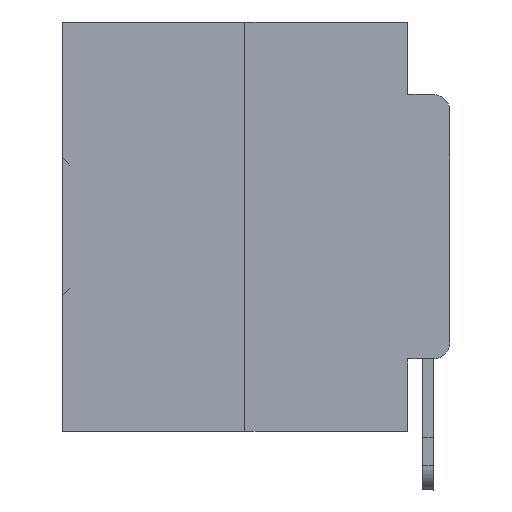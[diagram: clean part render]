
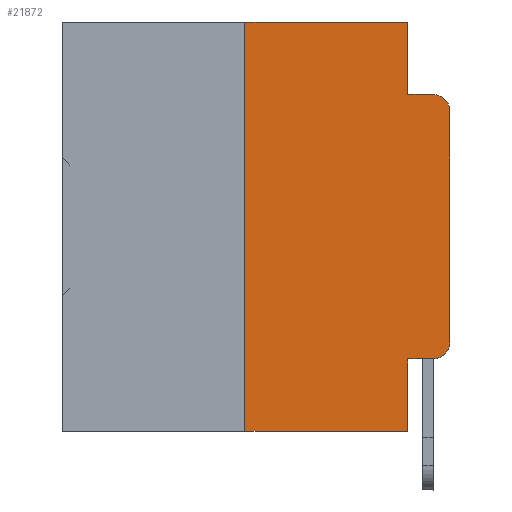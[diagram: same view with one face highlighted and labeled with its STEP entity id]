
A CAD part, left-side view. The second image highlights one B-rep face of the part: STEP entity #21872.
In plain terms, the highlighted planar face has unit normal (-1, 0, 0).
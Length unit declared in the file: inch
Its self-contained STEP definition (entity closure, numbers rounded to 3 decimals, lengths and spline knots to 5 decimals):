
#18 = CARTESIAN_POINT ( 'NONE',  ( 0., 0.473, 0. ) ) ;
#63 = VERTEX_POINT ( 'NONE', #4339 ) ;
#157 = VERTEX_POINT ( 'NONE', #22633 ) ;
#302 = CARTESIAN_POINT ( 'NONE',  ( 0., 0.051, -0.4115 ) ) ;
#1550 = CARTESIAN_POINT ( 'NONE',  ( 0., 0.02, -0.0885 ) ) ;
#1629 = ORIENTED_EDGE ( 'NONE', *, *, #2561, .F. ) ;
#1844 = CARTESIAN_POINT ( 'NONE',  ( 0., 0.25, 0. ) ) ;
#2561 = EDGE_CURVE ( 'NONE', #28601, #8657, #36051, .T. ) ;
#3637 = DIRECTION ( 'NONE',  ( 0., 0., -1. ) ) ;
#3762 = CARTESIAN_POINT ( 'NONE',  ( 0., 0.473, 0. ) ) ;
#4111 = DIRECTION ( 'NONE',  ( -1., 0., 0. ) ) ;
#4194 = EDGE_LOOP ( 'NONE', ( #5276, #21446, #27600, #12040, #25809, #35037, #9537, #1629, #8975, #7674 ) ) ;
#4339 = CARTESIAN_POINT ( 'NONE',  ( 0., 0.25, -0.5 ) ) ;
#5276 = ORIENTED_EDGE ( 'NONE', *, *, #27083, .T. ) ;
#5367 = DIRECTION ( 'NONE',  ( 0., -1., 0. ) ) ;
#5375 = CARTESIAN_POINT ( 'NONE',  ( 0., 0.25, 0. ) ) ;
#5873 = EDGE_CURVE ( 'NONE', #63, #8657, #11171, .T. ) ;
#6385 = LINE ( 'NONE', #6777, #14290 ) ;
#6777 = CARTESIAN_POINT ( 'NONE',  ( 0., 0., 0. ) ) ;
#7314 = AXIS2_PLACEMENT_3D ( 'NONE', #29098, #4111, #29586 ) ;
#7674 = ORIENTED_EDGE ( 'NONE', *, *, #22962, .T. ) ;
#8657 = VERTEX_POINT ( 'NONE', #8992 ) ;
#8975 = ORIENTED_EDGE ( 'NONE', *, *, #23795, .T. ) ;
#8992 = CARTESIAN_POINT ( 'NONE',  ( 0., 0.051, -0.5 ) ) ;
#8997 = CARTESIAN_POINT ( 'NONE',  ( 0., 0., -0.1085 ) ) ;
#9537 = ORIENTED_EDGE ( 'NONE', *, *, #5873, .T. ) ;
#10629 = DIRECTION ( 'NONE',  ( 0., 0., 1. ) ) ;
#10642 = CIRCLE ( 'NONE', #7314, 0.02 ) ;
#10894 = CARTESIAN_POINT ( 'NONE',  ( 0., 0.051, -0.0885 ) ) ;
#11163 = EDGE_CURVE ( 'NONE', #25966, #18093, #23819, .T. ) ;
#11171 = LINE ( 'NONE', #36032, #31705 ) ;
#11412 = LINE ( 'NONE', #34351, #13232 ) ;
#11983 = DIRECTION ( 'NONE',  ( 1., 0., 0. ) ) ;
#12040 = ORIENTED_EDGE ( 'NONE', *, *, #25967, .F. ) ;
#12396 = DIRECTION ( 'NONE',  ( 0., 0., -1. ) ) ;
#12795 = VERTEX_POINT ( 'NONE', #1844 ) ;
#13130 = EDGE_CURVE ( 'NONE', #22803, #18093, #18063, .T. ) ;
#13232 = VECTOR ( 'NONE', #20188, 39.37008 ) ;
#14215 = CARTESIAN_POINT ( 'NONE',  ( 0., 0.051, 0. ) ) ;
#14290 = VECTOR ( 'NONE', #26355, 39.37008 ) ;
#14361 = DIRECTION ( 'NONE',  ( 0., 0., -1. ) ) ;
#15394 = CARTESIAN_POINT ( 'NONE',  ( 0., 0.051, -0.0885 ) ) ;
#15781 = AXIS2_PLACEMENT_3D ( 'NONE', #3762, #11983, #3637 ) ;
#16267 = VECTOR ( 'NONE', #10629, 39.37008 ) ;
#16966 = VERTEX_POINT ( 'NONE', #14215 ) ;
#17629 = PLANE ( 'NONE',  #15781 ) ;
#18063 = CIRCLE ( 'NONE', #31660, 0.02 ) ;
#18093 = VERTEX_POINT ( 'NONE', #1550 ) ;
#18343 = VECTOR ( 'NONE', #14361, 39.37008 ) ;
#19301 = FACE_OUTER_BOUND ( 'NONE', #4194, .T. ) ;
#19600 = DIRECTION ( 'NONE',  ( 0., -1., 0. ) ) ;
#20188 = DIRECTION ( 'NONE',  ( 0., -1., 0. ) ) ;
#21446 = ORIENTED_EDGE ( 'NONE', *, *, #13130, .T. ) ;
#21872 = ADVANCED_FACE ( 'NONE', ( #19301 ), #17629, .F. ) ;
#22633 = CARTESIAN_POINT ( 'NONE',  ( 0., 0.02, -0.4115 ) ) ;
#22803 = VERTEX_POINT ( 'NONE', #8997 ) ;
#22962 = EDGE_CURVE ( 'NONE', #157, #32627, #10642, .T. ) ;
#23795 = EDGE_CURVE ( 'NONE', #28601, #157, #11412, .T. ) ;
#23819 = LINE ( 'NONE', #10894, #25558 ) ;
#25558 = VECTOR ( 'NONE', #35691, 39.37008 ) ;
#25809 = ORIENTED_EDGE ( 'NONE', *, *, #31632, .F. ) ;
#25966 = VERTEX_POINT ( 'NONE', #15394 ) ;
#25967 = EDGE_CURVE ( 'NONE', #16966, #25966, #28365, .T. ) ;
#26355 = DIRECTION ( 'NONE',  ( 0., 0., 1. ) ) ;
#27083 = EDGE_CURVE ( 'NONE', #32627, #22803, #6385, .T. ) ;
#27600 = ORIENTED_EDGE ( 'NONE', *, *, #11163, .F. ) ;
#28364 = CARTESIAN_POINT ( 'NONE',  ( 0., 0.02, -0.1085 ) ) ;
#28365 = LINE ( 'NONE', #34264, #18343 ) ;
#28475 = DIRECTION ( 'NONE',  ( 0., 0., -1. ) ) ;
#28601 = VERTEX_POINT ( 'NONE', #302 ) ;
#29098 = CARTESIAN_POINT ( 'NONE',  ( 0., 0.02, -0.3915 ) ) ;
#29272 = CARTESIAN_POINT ( 'NONE',  ( 0., 0.051, 0. ) ) ;
#29511 = VECTOR ( 'NONE', #12396, 39.37008 ) ;
#29586 = DIRECTION ( 'NONE',  ( 0., 0., -1. ) ) ;
#31632 = EDGE_CURVE ( 'NONE', #12795, #16966, #34122, .T. ) ;
#31660 = AXIS2_PLACEMENT_3D ( 'NONE', #28364, #34180, #28475 ) ;
#31705 = VECTOR ( 'NONE', #5367, 39.37008 ) ;
#31845 = CARTESIAN_POINT ( 'NONE',  ( 0., 0., -0.3915 ) ) ;
#32183 = EDGE_CURVE ( 'NONE', #63, #12795, #32840, .T. ) ;
#32627 = VERTEX_POINT ( 'NONE', #31845 ) ;
#32840 = LINE ( 'NONE', #5375, #16267 ) ;
#34122 = LINE ( 'NONE', #18, #35479 ) ;
#34180 = DIRECTION ( 'NONE',  ( -1., 0., 0. ) ) ;
#34264 = CARTESIAN_POINT ( 'NONE',  ( 0., 0.051, 0. ) ) ;
#34351 = CARTESIAN_POINT ( 'NONE',  ( 0., 0.051, -0.4115 ) ) ;
#35037 = ORIENTED_EDGE ( 'NONE', *, *, #32183, .F. ) ;
#35479 = VECTOR ( 'NONE', #19600, 39.37008 ) ;
#35691 = DIRECTION ( 'NONE',  ( 0., -1., 0. ) ) ;
#36032 = CARTESIAN_POINT ( 'NONE',  ( 0., 0.473, -0.5 ) ) ;
#36051 = LINE ( 'NONE', #29272, #29511 ) ;
